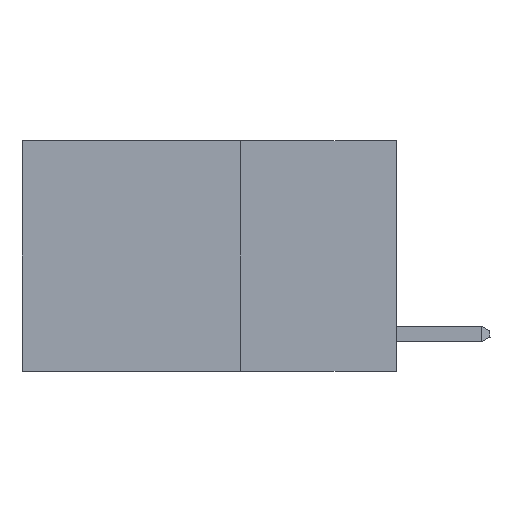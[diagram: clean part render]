
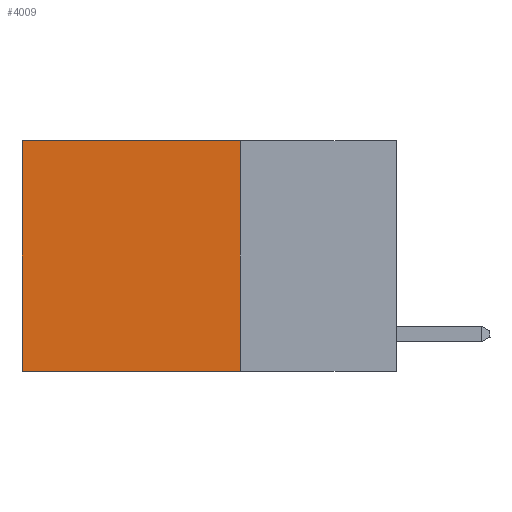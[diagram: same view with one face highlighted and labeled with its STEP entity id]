
A CAD part, left-side view. The second image highlights one B-rep face of the part: STEP entity #4009.
In plain terms, the highlighted planar face has unit normal (-1, 0, 0).
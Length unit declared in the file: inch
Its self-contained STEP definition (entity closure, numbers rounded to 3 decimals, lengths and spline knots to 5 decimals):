
#59 = EDGE_CURVE ( 'NONE', #610, #5758, #1249, .T. ) ;
#138 = PLANE ( 'NONE',  #3462 ) ;
#172 = CARTESIAN_POINT ( 'NONE',  ( 0.2625, 0.25, 0. ) ) ;
#437 = LINE ( 'NONE', #2692, #4255 ) ;
#610 = VERTEX_POINT ( 'NONE', #8069 ) ;
#740 = EDGE_CURVE ( 'NONE', #7305, #2656, #7102, .T. ) ;
#959 = DIRECTION ( 'NONE',  ( 1., 0., 0. ) ) ;
#1249 = LINE ( 'NONE', #2807, #8799 ) ;
#1610 = FACE_OUTER_BOUND ( 'NONE', #5309, .T. ) ;
#2063 = CARTESIAN_POINT ( 'NONE',  ( 0.2625, 0.6, 0. ) ) ;
#2120 = LINE ( 'NONE', #3677, #3875 ) ;
#2202 = CARTESIAN_POINT ( 'NONE',  ( 0.2625, 0.25, -0.37 ) ) ;
#2613 = EDGE_CURVE ( 'NONE', #610, #7305, #2120, .T. ) ;
#2656 = VERTEX_POINT ( 'NONE', #9750 ) ;
#2692 = CARTESIAN_POINT ( 'NONE',  ( 0.2625, 0.6, 0. ) ) ;
#2807 = CARTESIAN_POINT ( 'NONE',  ( 0.2625, 0.25, 0. ) ) ;
#2951 = ORIENTED_EDGE ( 'NONE', *, *, #59, .T. ) ;
#3204 = CARTESIAN_POINT ( 'NONE',  ( 0.2625, 0.25, -0.37 ) ) ;
#3462 = AXIS2_PLACEMENT_3D ( 'NONE', #172, #959, #6204 ) ;
#3677 = CARTESIAN_POINT ( 'NONE',  ( 0.2625, 0.25, 0. ) ) ;
#3875 = VECTOR ( 'NONE', #5171, 39.37008 ) ;
#4009 = ADVANCED_FACE ( 'NONE', ( #1610 ), #138, .F. ) ;
#4132 = ORIENTED_EDGE ( 'NONE', *, *, #740, .F. ) ;
#4255 = VECTOR ( 'NONE', #4969, 39.37008 ) ;
#4969 = DIRECTION ( 'NONE',  ( 0., 0., -1. ) ) ;
#5130 = VECTOR ( 'NONE', #9720, 39.37008 ) ;
#5171 = DIRECTION ( 'NONE',  ( 0., 0., -1. ) ) ;
#5309 = EDGE_LOOP ( 'NONE', ( #7487, #4132, #9738, #2951 ) ) ;
#5758 = VERTEX_POINT ( 'NONE', #2063 ) ;
#6204 = DIRECTION ( 'NONE',  ( 0., 0., -1. ) ) ;
#7102 = LINE ( 'NONE', #2202, #5130 ) ;
#7305 = VERTEX_POINT ( 'NONE', #3204 ) ;
#7487 = ORIENTED_EDGE ( 'NONE', *, *, #7573, .T. ) ;
#7573 = EDGE_CURVE ( 'NONE', #5758, #2656, #437, .T. ) ;
#8044 = DIRECTION ( 'NONE',  ( 0., 1., 0. ) ) ;
#8069 = CARTESIAN_POINT ( 'NONE',  ( 0.2625, 0.25, 0. ) ) ;
#8799 = VECTOR ( 'NONE', #8044, 39.37008 ) ;
#9720 = DIRECTION ( 'NONE',  ( 0., 1., 0. ) ) ;
#9738 = ORIENTED_EDGE ( 'NONE', *, *, #2613, .F. ) ;
#9750 = CARTESIAN_POINT ( 'NONE',  ( 0.2625, 0.6, -0.37 ) ) ;
